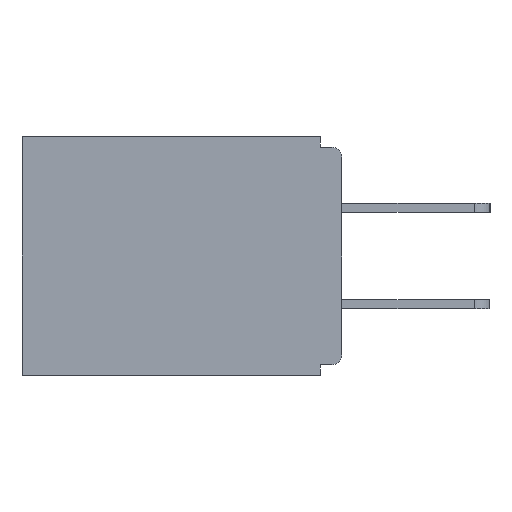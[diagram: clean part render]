
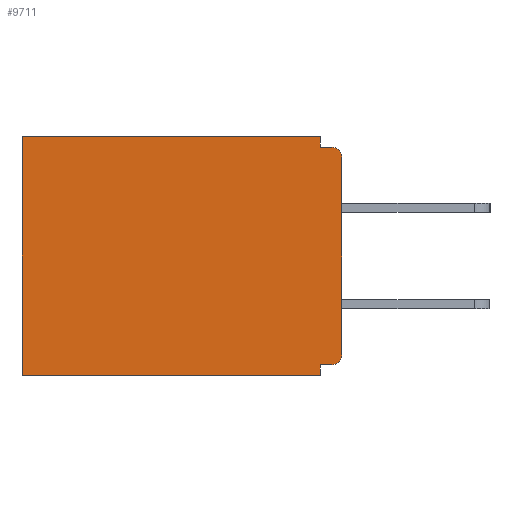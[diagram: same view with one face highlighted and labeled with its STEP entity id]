
A CAD part, left-side view. The second image highlights one B-rep face of the part: STEP entity #9711.
In plain terms, the highlighted planar face has unit normal (-1, 0, 0).
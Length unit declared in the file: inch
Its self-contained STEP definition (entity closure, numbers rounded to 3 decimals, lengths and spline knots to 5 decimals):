
#102 = EDGE_CURVE ( 'NONE', #9738, #8128, #3748, .T. ) ;
#159 = CARTESIAN_POINT ( 'NONE',  ( 0.298, 0., -0.015 ) ) ;
#189 = LINE ( 'NONE', #2169, #11440 ) ;
#268 = CARTESIAN_POINT ( 'NONE',  ( 0.298, 0.031, -0.343 ) ) ;
#280 = DIRECTION ( 'NONE',  ( 0., 0., -1. ) ) ;
#303 = CARTESIAN_POINT ( 'NONE',  ( 0.298, 0.031, -0.015 ) ) ;
#318 = DIRECTION ( 'NONE',  ( 0., 0., -1. ) ) ;
#1217 = CARTESIAN_POINT ( 'NONE',  ( 0.298, 0.46, 0. ) ) ;
#1422 = CARTESIAN_POINT ( 'NONE',  ( 0.298, 0.015, -0.03 ) ) ;
#1464 = CARTESIAN_POINT ( 'NONE',  ( 0.298, 0., -0.313 ) ) ;
#1521 = PLANE ( 'NONE',  #7556 ) ;
#1980 = LINE ( 'NONE', #4157, #9347 ) ;
#2082 = CIRCLE ( 'NONE', #6655, 0.015 ) ;
#2115 = EDGE_CURVE ( 'NONE', #8128, #11495, #7890, .T. ) ;
#2169 = CARTESIAN_POINT ( 'NONE',  ( 0.298, 0., 0. ) ) ;
#2250 = DIRECTION ( 'NONE',  ( -1., 0., 0. ) ) ;
#2813 = LINE ( 'NONE', #159, #10317 ) ;
#3137 = EDGE_CURVE ( 'NONE', #11515, #3370, #189, .T. ) ;
#3317 = DIRECTION ( 'NONE',  ( 1., 0., 0. ) ) ;
#3370 = VERTEX_POINT ( 'NONE', #1464 ) ;
#3387 = CARTESIAN_POINT ( 'NONE',  ( 0.298, 0.46, 0. ) ) ;
#3437 = CARTESIAN_POINT ( 'NONE',  ( 0.298, 0., 0. ) ) ;
#3476 = EDGE_CURVE ( 'NONE', #7213, #3602, #4645, .T. ) ;
#3602 = VERTEX_POINT ( 'NONE', #303 ) ;
#3748 = LINE ( 'NONE', #9333, #11213 ) ;
#3912 = DIRECTION ( 'NONE',  ( 0., -1., 0. ) ) ;
#4157 = CARTESIAN_POINT ( 'NONE',  ( 0.298, 0., -0.343 ) ) ;
#4251 = EDGE_CURVE ( 'NONE', #11515, #8190, #2082, .T. ) ;
#4418 = EDGE_CURVE ( 'NONE', #7213, #8652, #7212, .T. ) ;
#4445 = VECTOR ( 'NONE', #318, 39.37008 ) ;
#4584 = CARTESIAN_POINT ( 'NONE',  ( 0.298, 0.46, -0.343 ) ) ;
#4645 = LINE ( 'NONE', #268, #8827 ) ;
#4846 = VECTOR ( 'NONE', #11742, 39.37008 ) ;
#5149 = ORIENTED_EDGE ( 'NONE', *, *, #3476, .F. ) ;
#5286 = DIRECTION ( 'NONE',  ( 0., 0., -1. ) ) ;
#5310 = FACE_OUTER_BOUND ( 'NONE', #11842, .T. ) ;
#5323 = DIRECTION ( 'NONE',  ( 0., 0., -1. ) ) ;
#5538 = DIRECTION ( 'NONE',  ( 0., 0., -1. ) ) ;
#5698 = CIRCLE ( 'NONE', #11391, 0.015 ) ;
#6132 = DIRECTION ( 'NONE',  ( 0., 1., 0. ) ) ;
#6206 = CARTESIAN_POINT ( 'NONE',  ( 0.298, 0.031, -0.343 ) ) ;
#6494 = DIRECTION ( 'NONE',  ( 0., 1., 0. ) ) ;
#6655 = AXIS2_PLACEMENT_3D ( 'NONE', #1422, #7607, #7843 ) ;
#6837 = EDGE_CURVE ( 'NONE', #3602, #8190, #2813, .T. ) ;
#6967 = VECTOR ( 'NONE', #5538, 39.37008 ) ;
#7097 = CARTESIAN_POINT ( 'NONE',  ( 0.298, 0.015, -0.313 ) ) ;
#7116 = CARTESIAN_POINT ( 'NONE',  ( 0.298, 0., 0. ) ) ;
#7212 = LINE ( 'NONE', #7116, #4846 ) ;
#7213 = VERTEX_POINT ( 'NONE', #7703 ) ;
#7253 = CARTESIAN_POINT ( 'NONE',  ( 0.298, 0.031, -0.343 ) ) ;
#7393 = EDGE_CURVE ( 'NONE', #9738, #3370, #5698, .T. ) ;
#7429 = ORIENTED_EDGE ( 'NONE', *, *, #6837, .F. ) ;
#7556 = AXIS2_PLACEMENT_3D ( 'NONE', #3437, #3317, #5286 ) ;
#7607 = DIRECTION ( 'NONE',  ( -1., 0., 0. ) ) ;
#7689 = VERTEX_POINT ( 'NONE', #4584 ) ;
#7703 = CARTESIAN_POINT ( 'NONE',  ( 0.298, 0.031, 0. ) ) ;
#7843 = DIRECTION ( 'NONE',  ( 0., 0., -1. ) ) ;
#7890 = LINE ( 'NONE', #6206, #4445 ) ;
#8128 = VERTEX_POINT ( 'NONE', #9947 ) ;
#8150 = CARTESIAN_POINT ( 'NONE',  ( 0.298, 0.015, -0.328 ) ) ;
#8190 = VERTEX_POINT ( 'NONE', #10232 ) ;
#8652 = VERTEX_POINT ( 'NONE', #1217 ) ;
#8827 = VECTOR ( 'NONE', #9828, 39.37008 ) ;
#8940 = CARTESIAN_POINT ( 'NONE',  ( 0.298, 0., -0.03 ) ) ;
#9076 = LINE ( 'NONE', #3387, #6967 ) ;
#9148 = ORIENTED_EDGE ( 'NONE', *, *, #4251, .T. ) ;
#9333 = CARTESIAN_POINT ( 'NONE',  ( 0.298, 0., -0.328 ) ) ;
#9347 = VECTOR ( 'NONE', #6132, 39.37008 ) ;
#9438 = ORIENTED_EDGE ( 'NONE', *, *, #2115, .F. ) ;
#9595 = ORIENTED_EDGE ( 'NONE', *, *, #7393, .T. ) ;
#9711 = ADVANCED_FACE ( 'NONE', ( #5310 ), #1521, .F. ) ;
#9738 = VERTEX_POINT ( 'NONE', #8150 ) ;
#9828 = DIRECTION ( 'NONE',  ( 0., 0., -1. ) ) ;
#9947 = CARTESIAN_POINT ( 'NONE',  ( 0.298, 0.031, -0.328 ) ) ;
#10124 = ORIENTED_EDGE ( 'NONE', *, *, #3137, .F. ) ;
#10232 = CARTESIAN_POINT ( 'NONE',  ( 0.298, 0.015, -0.015 ) ) ;
#10317 = VECTOR ( 'NONE', #3912, 39.37008 ) ;
#10418 = ORIENTED_EDGE ( 'NONE', *, *, #11830, .F. ) ;
#11178 = EDGE_CURVE ( 'NONE', #8652, #7689, #9076, .T. ) ;
#11197 = ORIENTED_EDGE ( 'NONE', *, *, #4418, .T. ) ;
#11213 = VECTOR ( 'NONE', #6494, 39.37008 ) ;
#11391 = AXIS2_PLACEMENT_3D ( 'NONE', #7097, #2250, #280 ) ;
#11440 = VECTOR ( 'NONE', #5323, 39.37008 ) ;
#11495 = VERTEX_POINT ( 'NONE', #7253 ) ;
#11515 = VERTEX_POINT ( 'NONE', #8940 ) ;
#11536 = ORIENTED_EDGE ( 'NONE', *, *, #102, .F. ) ;
#11742 = DIRECTION ( 'NONE',  ( 0., 1., 0. ) ) ;
#11830 = EDGE_CURVE ( 'NONE', #11495, #7689, #1980, .T. ) ;
#11842 = EDGE_LOOP ( 'NONE', ( #9148, #7429, #5149, #11197, #12331, #10418, #9438, #11536, #9595, #10124 ) ) ;
#12331 = ORIENTED_EDGE ( 'NONE', *, *, #11178, .T. ) ;
